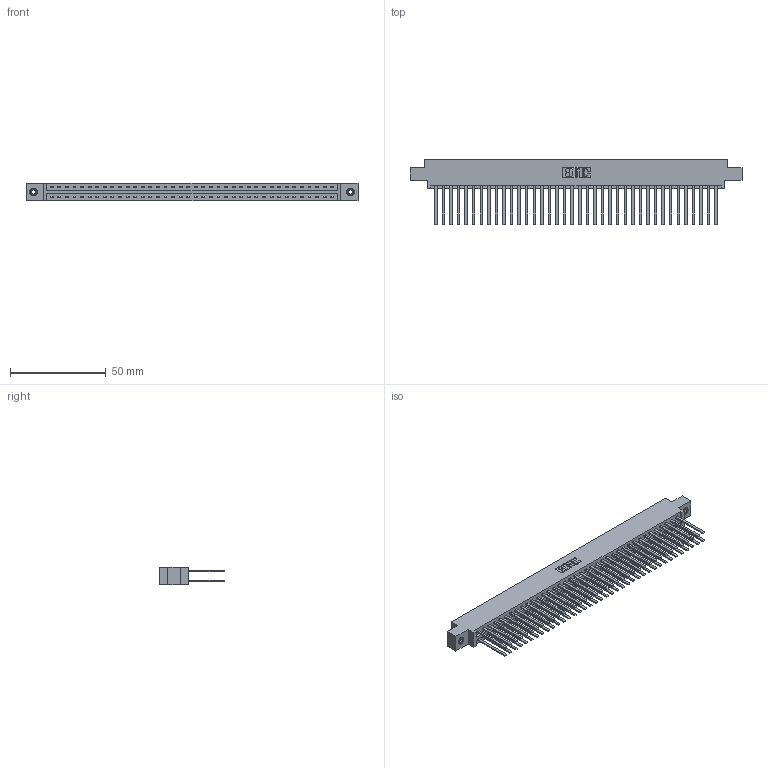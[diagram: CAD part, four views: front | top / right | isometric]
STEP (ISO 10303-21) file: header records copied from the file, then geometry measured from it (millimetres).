
FILE_DESCRIPTION (( 'STEP AP203' ), '1' );
FILE_NAME ('387-076-544-808.STEP', '2018-09-23T15:57:51', ( '' ), ( '' ), 'SwSTEP 2.0', 'SolidWorks 2016', '' );
FILE_SCHEMA (( 'CONFIG_CONTROL_DESIGN' ));
Length unit declared in the file: inch
Products named in the file (4): 387-076-544-808; 337 Part_0.170 Offset - 0.156 Dia-TI; 345-292-001_345-293-144; 345-250-001_345-250-003-102
Assembly tree (79 placements, depth 2):
  387-076-544-808
    337 Part_0.170 Offset - 0.156 Dia-TI
    345-292-001_345-293-144  x76
    345-250-001_345-250-003-102  x2
Bounding box: 173.58 x 34.3 x 9.4 mm (x, y, z)
Volume: 19181.7 mm3; surface area: 25258.2 mm2
Topology: 79 solids, 79 shells, 3826 faces, 11327 edges, 7442 vertices
Faces by surface type: plane 2690, cylinder 1120, cone 12, torus 4
Entity records: 31114 total; most frequent: CARTESIAN_POINT 5225, ORIENTED_EDGE 5154, DIRECTION 4479, EDGE_CURVE 2577, LINE 2433, VECTOR 2433, VERTEX_POINT 1712, AXIS2_PLACEMENT_3D 1023
